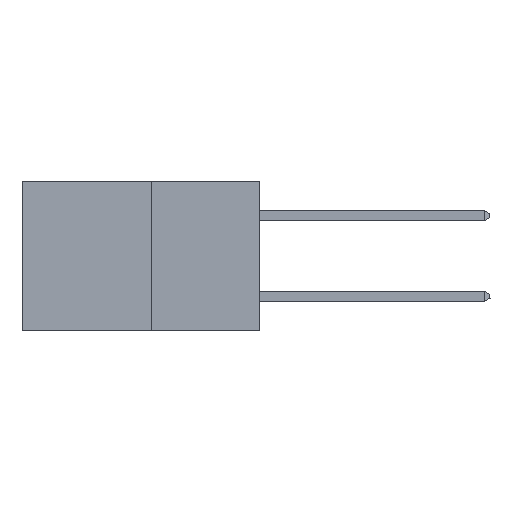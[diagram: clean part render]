
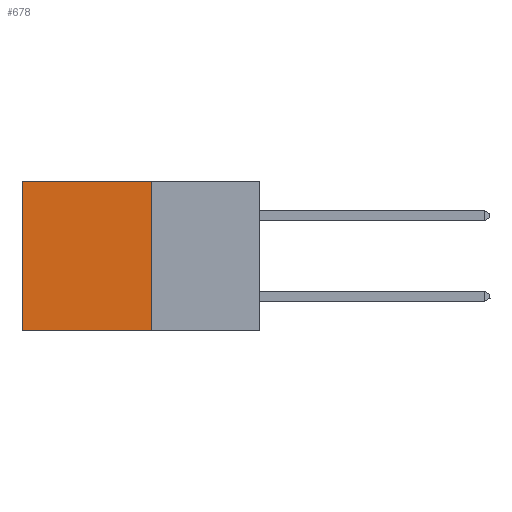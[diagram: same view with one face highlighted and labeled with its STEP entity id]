
A CAD part, left-side view. The second image highlights one B-rep face of the part: STEP entity #678.
In plain terms, the highlighted planar face has unit normal (-1, 0, 0).
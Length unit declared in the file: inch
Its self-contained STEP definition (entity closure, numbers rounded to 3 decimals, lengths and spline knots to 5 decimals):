
#202 = AXIS2_PLACEMENT_3D ( 'NONE', #22477, #2450, #20048 ) ;
#678 = ADVANCED_FACE ( 'NONE', ( #12923 ), #18163, .F. ) ;
#1393 = VECTOR ( 'NONE', #8058, 39.37008 ) ;
#2450 = DIRECTION ( 'NONE',  ( 1., 0., 0. ) ) ;
#2928 = LINE ( 'NONE', #18350, #12007 ) ;
#2934 = VERTEX_POINT ( 'NONE', #5586 ) ;
#3950 = ORIENTED_EDGE ( 'NONE', *, *, #17823, .F. ) ;
#5586 = CARTESIAN_POINT ( 'NONE',  ( 0.277, 0.59, -0.37 ) ) ;
#5843 = VECTOR ( 'NONE', #18426, 39.37008 ) ;
#6221 = CARTESIAN_POINT ( 'NONE',  ( 0.277, 0.27, -0.37 ) ) ;
#6730 = VECTOR ( 'NONE', #22805, 39.37008 ) ;
#7676 = VERTEX_POINT ( 'NONE', #18814 ) ;
#8058 = DIRECTION ( 'NONE',  ( 0., 0., -1. ) ) ;
#8383 = ORIENTED_EDGE ( 'NONE', *, *, #14747, .F. ) ;
#9954 = ORIENTED_EDGE ( 'NONE', *, *, #16110, .T. ) ;
#10664 = EDGE_CURVE ( 'NONE', #20623, #7676, #20286, .T. ) ;
#10963 = LINE ( 'NONE', #13754, #6730 ) ;
#12007 = VECTOR ( 'NONE', #20163, 39.37008 ) ;
#12533 = ORIENTED_EDGE ( 'NONE', *, *, #10664, .T. ) ;
#12923 = FACE_OUTER_BOUND ( 'NONE', #17911, .T. ) ;
#12958 = CARTESIAN_POINT ( 'NONE',  ( 0.277, 0.27, 0. ) ) ;
#13754 = CARTESIAN_POINT ( 'NONE',  ( 0.277, 0.59, -0.37 ) ) ;
#14747 = EDGE_CURVE ( 'NONE', #20623, #15840, #15819, .T. ) ;
#15819 = LINE ( 'NONE', #6221, #1393 ) ;
#15840 = VERTEX_POINT ( 'NONE', #22028 ) ;
#16110 = EDGE_CURVE ( 'NONE', #7676, #2934, #10963, .T. ) ;
#17823 = EDGE_CURVE ( 'NONE', #15840, #2934, #2928, .T. ) ;
#17911 = EDGE_LOOP ( 'NONE', ( #9954, #3950, #8383, #12533 ) ) ;
#18163 = PLANE ( 'NONE',  #202 ) ;
#18350 = CARTESIAN_POINT ( 'NONE',  ( 0.277, 0.27, -0.37 ) ) ;
#18426 = DIRECTION ( 'NONE',  ( 0., 1., 0. ) ) ;
#18814 = CARTESIAN_POINT ( 'NONE',  ( 0.277, 0.59, 0. ) ) ;
#20048 = DIRECTION ( 'NONE',  ( 0., 0., -1. ) ) ;
#20163 = DIRECTION ( 'NONE',  ( 0., 1., 0. ) ) ;
#20286 = LINE ( 'NONE', #12958, #5843 ) ;
#20623 = VERTEX_POINT ( 'NONE', #21132 ) ;
#21132 = CARTESIAN_POINT ( 'NONE',  ( 0.277, 0.27, 0. ) ) ;
#22028 = CARTESIAN_POINT ( 'NONE',  ( 0.277, 0.27, -0.37 ) ) ;
#22477 = CARTESIAN_POINT ( 'NONE',  ( 0.277, 0.27, -0.37 ) ) ;
#22805 = DIRECTION ( 'NONE',  ( 0., 0., -1. ) ) ;
